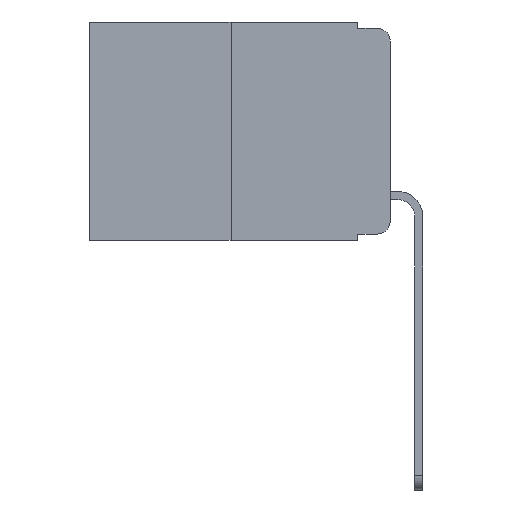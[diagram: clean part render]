
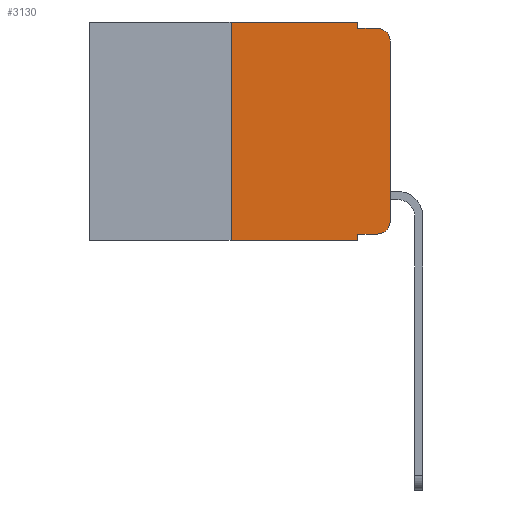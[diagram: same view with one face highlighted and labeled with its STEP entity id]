
A CAD part, left-side view. The second image highlights one B-rep face of the part: STEP entity #3130.
In plain terms, the highlighted planar face has unit normal (-1, 0, 0).
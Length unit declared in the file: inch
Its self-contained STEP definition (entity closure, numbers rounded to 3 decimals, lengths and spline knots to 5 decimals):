
#62 = DIRECTION ( 'NONE',  ( 0., -1., 0. ) ) ;
#146 = DIRECTION ( 'NONE',  ( 0., 0., -1. ) ) ;
#266 = VERTEX_POINT ( 'NONE', #1161 ) ;
#282 = VERTEX_POINT ( 'NONE', #11819 ) ;
#479 = DIRECTION ( 'NONE',  ( 0., 0., -1. ) ) ;
#543 = EDGE_CURVE ( 'NONE', #7029, #6240, #12846, .T. ) ;
#674 = VERTEX_POINT ( 'NONE', #14041 ) ;
#822 = VECTOR ( 'NONE', #6896, 39.37008 ) ;
#1161 = CARTESIAN_POINT ( 'NONE',  ( 0., 0.25, 0. ) ) ;
#1442 = LINE ( 'NONE', #1919, #7600 ) ;
#1749 = CARTESIAN_POINT ( 'NONE',  ( 0., 0.25, 0. ) ) ;
#1919 = CARTESIAN_POINT ( 'NONE',  ( 0., 0.051, -0.01 ) ) ;
#1926 = CARTESIAN_POINT ( 'NONE',  ( 0., 0.051, 0. ) ) ;
#2421 = VERTEX_POINT ( 'NONE', #5595 ) ;
#2477 = CARTESIAN_POINT ( 'NONE',  ( 0., 0., 0. ) ) ;
#2529 = EDGE_CURVE ( 'NONE', #7029, #674, #11126, .T. ) ;
#2578 = ORIENTED_EDGE ( 'NONE', *, *, #7677, .T. ) ;
#2942 = VECTOR ( 'NONE', #62, 39.37008 ) ;
#3130 = ADVANCED_FACE ( 'NONE', ( #10183 ), #8011, .F. ) ;
#3366 = DIRECTION ( 'NONE',  ( 0., -1., 0. ) ) ;
#3497 = EDGE_CURVE ( 'NONE', #13136, #266, #5069, .T. ) ;
#3522 = LINE ( 'NONE', #10412, #9006 ) ;
#3685 = VECTOR ( 'NONE', #14915, 39.37008 ) ;
#3880 = CARTESIAN_POINT ( 'NONE',  ( 0., 0.051, -0.333 ) ) ;
#4398 = CARTESIAN_POINT ( 'NONE',  ( 0., 0.473, 0. ) ) ;
#4547 = DIRECTION ( 'NONE',  ( -1., 0., 0. ) ) ;
#5069 = LINE ( 'NONE', #1749, #11270 ) ;
#5414 = EDGE_LOOP ( 'NONE', ( #5973, #2578, #15311, #13187, #11575, #10186, #10599, #9258, #11051, #11769 ) ) ;
#5595 = CARTESIAN_POINT ( 'NONE',  ( 0., 0.051, -0.01 ) ) ;
#5973 = ORIENTED_EDGE ( 'NONE', *, *, #9376, .T. ) ;
#6023 = EDGE_CURVE ( 'NONE', #10764, #2421, #3522, .T. ) ;
#6240 = VERTEX_POINT ( 'NONE', #7945 ) ;
#6468 = CARTESIAN_POINT ( 'NONE',  ( 0., 0.473, -0.343 ) ) ;
#6519 = LINE ( 'NONE', #2477, #13398 ) ;
#6802 = DIRECTION ( 'NONE',  ( -1., 0., 0. ) ) ;
#6837 = EDGE_CURVE ( 'NONE', #2421, #282, #1442, .T. ) ;
#6896 = DIRECTION ( 'NONE',  ( 0., -1., 0. ) ) ;
#7029 = VERTEX_POINT ( 'NONE', #3880 ) ;
#7064 = EDGE_CURVE ( 'NONE', #13136, #674, #16156, .T. ) ;
#7521 = DIRECTION ( 'NONE',  ( 0., 0., 1. ) ) ;
#7600 = VECTOR ( 'NONE', #3366, 39.37008 ) ;
#7667 = VERTEX_POINT ( 'NONE', #11897 ) ;
#7677 = EDGE_CURVE ( 'NONE', #7667, #282, #8161, .T. ) ;
#7945 = CARTESIAN_POINT ( 'NONE',  ( 0., 0.02, -0.333 ) ) ;
#8011 = PLANE ( 'NONE',  #9500 ) ;
#8161 = CIRCLE ( 'NONE', #8824, 0.02 ) ;
#8824 = AXIS2_PLACEMENT_3D ( 'NONE', #11942, #4547, #13137 ) ;
#8850 = CARTESIAN_POINT ( 'NONE',  ( 0., 0.051, -0.333 ) ) ;
#9006 = VECTOR ( 'NONE', #9174, 39.37008 ) ;
#9025 = CARTESIAN_POINT ( 'NONE',  ( 0., 0.473, 0. ) ) ;
#9174 = DIRECTION ( 'NONE',  ( 0., 0., -1. ) ) ;
#9258 = ORIENTED_EDGE ( 'NONE', *, *, #2529, .F. ) ;
#9376 = EDGE_CURVE ( 'NONE', #14546, #7667, #6519, .T. ) ;
#9500 = AXIS2_PLACEMENT_3D ( 'NONE', #9025, #13596, #146 ) ;
#9851 = CARTESIAN_POINT ( 'NONE',  ( 0., 0.051, 0. ) ) ;
#10153 = AXIS2_PLACEMENT_3D ( 'NONE', #14076, #6802, #15231 ) ;
#10183 = FACE_OUTER_BOUND ( 'NONE', #5414, .T. ) ;
#10186 = ORIENTED_EDGE ( 'NONE', *, *, #3497, .F. ) ;
#10412 = CARTESIAN_POINT ( 'NONE',  ( 0., 0.051, 0. ) ) ;
#10587 = CARTESIAN_POINT ( 'NONE',  ( 0., 0., -0.313 ) ) ;
#10599 = ORIENTED_EDGE ( 'NONE', *, *, #7064, .T. ) ;
#10764 = VERTEX_POINT ( 'NONE', #1926 ) ;
#11051 = ORIENTED_EDGE ( 'NONE', *, *, #543, .T. ) ;
#11126 = LINE ( 'NONE', #9851, #13869 ) ;
#11159 = LINE ( 'NONE', #4398, #822 ) ;
#11270 = VECTOR ( 'NONE', #7521, 39.37008 ) ;
#11575 = ORIENTED_EDGE ( 'NONE', *, *, #14586, .F. ) ;
#11769 = ORIENTED_EDGE ( 'NONE', *, *, #15970, .T. ) ;
#11819 = CARTESIAN_POINT ( 'NONE',  ( 0., 0.02, -0.01 ) ) ;
#11897 = CARTESIAN_POINT ( 'NONE',  ( 0., 0., -0.03 ) ) ;
#11942 = CARTESIAN_POINT ( 'NONE',  ( 0., 0.02, -0.03 ) ) ;
#12582 = CIRCLE ( 'NONE', #10153, 0.02 ) ;
#12846 = LINE ( 'NONE', #8850, #2942 ) ;
#13136 = VERTEX_POINT ( 'NONE', #13243 ) ;
#13137 = DIRECTION ( 'NONE',  ( 0., 0., -1. ) ) ;
#13187 = ORIENTED_EDGE ( 'NONE', *, *, #6023, .F. ) ;
#13243 = CARTESIAN_POINT ( 'NONE',  ( 0., 0.25, -0.343 ) ) ;
#13398 = VECTOR ( 'NONE', #14782, 39.37008 ) ;
#13596 = DIRECTION ( 'NONE',  ( 1., 0., 0. ) ) ;
#13869 = VECTOR ( 'NONE', #479, 39.37008 ) ;
#14041 = CARTESIAN_POINT ( 'NONE',  ( 0., 0.051, -0.343 ) ) ;
#14076 = CARTESIAN_POINT ( 'NONE',  ( 0., 0.02, -0.313 ) ) ;
#14546 = VERTEX_POINT ( 'NONE', #10587 ) ;
#14586 = EDGE_CURVE ( 'NONE', #266, #10764, #11159, .T. ) ;
#14782 = DIRECTION ( 'NONE',  ( 0., 0., 1. ) ) ;
#14915 = DIRECTION ( 'NONE',  ( 0., -1., 0. ) ) ;
#15231 = DIRECTION ( 'NONE',  ( 0., 0., -1. ) ) ;
#15311 = ORIENTED_EDGE ( 'NONE', *, *, #6837, .F. ) ;
#15970 = EDGE_CURVE ( 'NONE', #6240, #14546, #12582, .T. ) ;
#16156 = LINE ( 'NONE', #6468, #3685 ) ;
